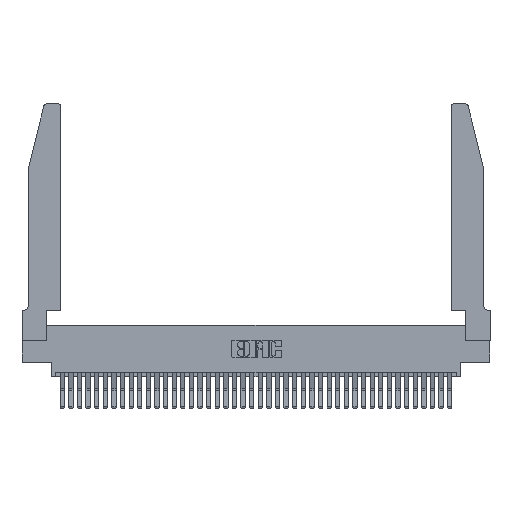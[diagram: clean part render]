
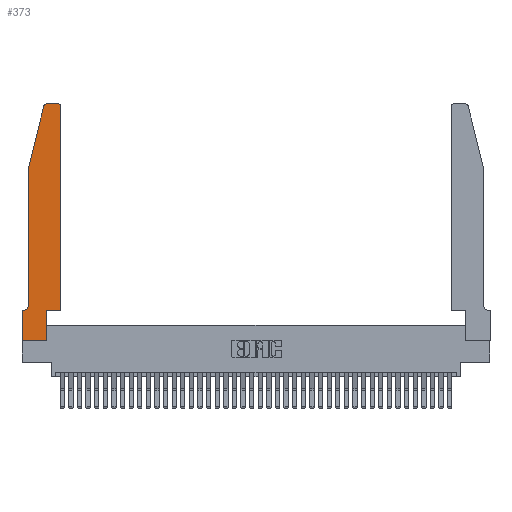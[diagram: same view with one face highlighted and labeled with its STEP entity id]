
A CAD part, top view. The second image highlights one B-rep face of the part: STEP entity #373.
In plain terms, the highlighted planar face has unit normal (0, 0, 1).
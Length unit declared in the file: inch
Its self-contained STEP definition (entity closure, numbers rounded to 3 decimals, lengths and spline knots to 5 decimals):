
#373 = ADVANCED_FACE ( 'NONE', ( #22306 ), #39974, .T. ) ;
#503 = DIRECTION ( 'NONE',  ( 0., 0., 1. ) ) ;
#1064 = ORIENTED_EDGE ( 'NONE', *, *, #20258, .T. ) ;
#1208 = AXIS2_PLACEMENT_3D ( 'NONE', #26135, #7357, #29238 ) ;
#1246 = EDGE_CURVE ( 'NONE', #1962, #23233, #16376, .T. ) ;
#1313 = CARTESIAN_POINT ( 'NONE',  ( 0.0755, 0.35, 0.37 ) ) ;
#1356 = EDGE_CURVE ( 'NONE', #24464, #34777, #13426, .T. ) ;
#1374 = DIRECTION ( 'NONE',  ( 0., 0., -1. ) ) ;
#1413 = EDGE_CURVE ( 'NONE', #3583, #27949, #17829, .T. ) ;
#1902 = VERTEX_POINT ( 'NONE', #19401 ) ;
#1962 = VERTEX_POINT ( 'NONE', #4251 ) ;
#2274 = LINE ( 'NONE', #35966, #11715 ) ;
#2526 = CARTESIAN_POINT ( 'NONE',  ( 0., 0.35, 0.37 ) ) ;
#3385 = CARTESIAN_POINT ( 'NONE',  ( 0.4205, 2.75, 0.37 ) ) ;
#3583 = VERTEX_POINT ( 'NONE', #28096 ) ;
#3814 = VERTEX_POINT ( 'NONE', #20504 ) ;
#4251 = CARTESIAN_POINT ( 'NONE',  ( 0.4505, 2.72, 0.37 ) ) ;
#4574 = EDGE_CURVE ( 'NONE', #27949, #27562, #8289, .T. ) ;
#4876 = VECTOR ( 'NONE', #6481, 39.37008 ) ;
#5573 = AXIS2_PLACEMENT_3D ( 'NONE', #20307, #1374, #23470 ) ;
#5749 = DIRECTION ( 'NONE',  ( 0., 0., 1. ) ) ;
#6366 = VECTOR ( 'NONE', #7573, 39.37008 ) ;
#6481 = DIRECTION ( 'NONE',  ( -0.239, -0.971, 0. ) ) ;
#6802 = VERTEX_POINT ( 'NONE', #23589 ) ;
#7245 = DIRECTION ( 'NONE',  ( 0., 1., 0. ) ) ;
#7311 = VECTOR ( 'NONE', #39691, 39.37008 ) ;
#7357 = DIRECTION ( 'NONE',  ( 0., 0., 1. ) ) ;
#7365 = LINE ( 'NONE', #20207, #6366 ) ;
#7573 = DIRECTION ( 'NONE',  ( -1., 0., 0. ) ) ;
#8111 = EDGE_CURVE ( 'NONE', #37173, #3814, #37953, .T. ) ;
#8289 = LINE ( 'NONE', #27271, #7311 ) ;
#9199 = CARTESIAN_POINT ( 'NONE',  ( 0.2865, 0.35, 0.37 ) ) ;
#9563 = ORIENTED_EDGE ( 'NONE', *, *, #8111, .T. ) ;
#9931 = CIRCLE ( 'NONE', #5573, 0.07 ) ;
#10021 = ORIENTED_EDGE ( 'NONE', *, *, #1356, .T. ) ;
#10969 = EDGE_CURVE ( 'NONE', #35680, #1962, #33832, .T. ) ;
#11715 = VECTOR ( 'NONE', #14183, 39.37008 ) ;
#12067 = EDGE_CURVE ( 'NONE', #34777, #1902, #19646, .T. ) ;
#12538 = CARTESIAN_POINT ( 'NONE',  ( 0.2865, 0., 0.37 ) ) ;
#12954 = VECTOR ( 'NONE', #15835, 39.37008 ) ;
#12986 = ORIENTED_EDGE ( 'NONE', *, *, #14734, .T. ) ;
#13120 = VECTOR ( 'NONE', #21284, 39.37008 ) ;
#13426 = CIRCLE ( 'NONE', #1208, 0.03 ) ;
#13847 = DIRECTION ( 'NONE',  ( 1., 0., 0. ) ) ;
#14183 = DIRECTION ( 'NONE',  ( 0., -1., 0. ) ) ;
#14216 = AXIS2_PLACEMENT_3D ( 'NONE', #2526, #5749, #27666 ) ;
#14734 = EDGE_CURVE ( 'NONE', #6802, #3583, #9931, .T. ) ;
#14781 = CARTESIAN_POINT ( 'NONE',  ( 0.284, 2.75, 0.37 ) ) ;
#15835 = DIRECTION ( 'NONE',  ( 1., 0., 0. ) ) ;
#15851 = CARTESIAN_POINT ( 'NONE',  ( 0.0755, 2., 0.37 ) ) ;
#16376 = CIRCLE ( 'NONE', #37693, 0.03 ) ;
#16624 = LINE ( 'NONE', #29404, #32203 ) ;
#16729 = CARTESIAN_POINT ( 'NONE',  ( 0.4505, 0.35, 0.37 ) ) ;
#17829 = LINE ( 'NONE', #1313, #26137 ) ;
#18476 = ORIENTED_EDGE ( 'NONE', *, *, #1246, .T. ) ;
#19401 = CARTESIAN_POINT ( 'NONE',  ( 0.0755, 2., 0.37 ) ) ;
#19414 = CARTESIAN_POINT ( 'NONE',  ( 0., 0., 0.37 ) ) ;
#19434 = CARTESIAN_POINT ( 'NONE',  ( 0.4205, 2.72, 0.37 ) ) ;
#19646 = LINE ( 'NONE', #15851, #4876 ) ;
#19858 = ORIENTED_EDGE ( 'NONE', *, *, #27042, .T. ) ;
#20207 = CARTESIAN_POINT ( 'NONE',  ( 0.2605, 2.75, 0.37 ) ) ;
#20258 = EDGE_CURVE ( 'NONE', #27562, #37173, #36812, .T. ) ;
#20307 = CARTESIAN_POINT ( 'NONE',  ( 0.0055, 0.42, 0.37 ) ) ;
#20334 = ORIENTED_EDGE ( 'NONE', *, *, #40394, .T. ) ;
#20504 = CARTESIAN_POINT ( 'NONE',  ( 0.2865, 0.35, 0.37 ) ) ;
#21284 = DIRECTION ( 'NONE',  ( 0., 1., 0. ) ) ;
#22306 = FACE_OUTER_BOUND ( 'NONE', #33698, .T. ) ;
#22613 = DIRECTION ( 'NONE',  ( 1., 0., 0. ) ) ;
#23233 = VERTEX_POINT ( 'NONE', #3385 ) ;
#23297 = ORIENTED_EDGE ( 'NONE', *, *, #1413, .T. ) ;
#23412 = DIRECTION ( 'NONE',  ( -1., 0., 0. ) ) ;
#23470 = DIRECTION ( 'NONE',  ( -1., 0., 0. ) ) ;
#23589 = CARTESIAN_POINT ( 'NONE',  ( 0.0755, 0.42, 0.37 ) ) ;
#23772 = ORIENTED_EDGE ( 'NONE', *, *, #32346, .T. ) ;
#24308 = CARTESIAN_POINT ( 'NONE',  ( 0.25487, 2.72718, 0.37 ) ) ;
#24464 = VERTEX_POINT ( 'NONE', #14781 ) ;
#26034 = CARTESIAN_POINT ( 'NONE',  ( 0.4505, 0.35, 0.37 ) ) ;
#26135 = CARTESIAN_POINT ( 'NONE',  ( 0.284, 2.72, 0.37 ) ) ;
#26137 = VECTOR ( 'NONE', #23412, 39.37008 ) ;
#26574 = VECTOR ( 'NONE', #7245, 39.37008 ) ;
#26670 = ORIENTED_EDGE ( 'NONE', *, *, #12067, .T. ) ;
#27042 = EDGE_CURVE ( 'NONE', #3814, #35680, #16624, .T. ) ;
#27271 = CARTESIAN_POINT ( 'NONE',  ( 0., 0., 0.37 ) ) ;
#27562 = VERTEX_POINT ( 'NONE', #19414 ) ;
#27666 = DIRECTION ( 'NONE',  ( 1., 0., 0. ) ) ;
#27949 = VERTEX_POINT ( 'NONE', #33385 ) ;
#28096 = CARTESIAN_POINT ( 'NONE',  ( 0.0055, 0.35, 0.37 ) ) ;
#28144 = ORIENTED_EDGE ( 'NONE', *, *, #10969, .T. ) ;
#29238 = DIRECTION ( 'NONE',  ( 1., 0., 0. ) ) ;
#29404 = CARTESIAN_POINT ( 'NONE',  ( 0.4505, 0.35, 0.37 ) ) ;
#32203 = VECTOR ( 'NONE', #13847, 39.37008 ) ;
#32346 = EDGE_CURVE ( 'NONE', #23233, #24464, #7365, .T. ) ;
#33385 = CARTESIAN_POINT ( 'NONE',  ( 0., 0.35, 0.37 ) ) ;
#33698 = EDGE_LOOP ( 'NONE', ( #23772, #10021, #26670, #20334, #12986, #23297, #39733, #1064, #9563, #19858, #28144, #18476 ) ) ;
#33832 = LINE ( 'NONE', #26034, #26574 ) ;
#34464 = CARTESIAN_POINT ( 'NONE',  ( 0., 0., 0.37 ) ) ;
#34777 = VERTEX_POINT ( 'NONE', #24308 ) ;
#35680 = VERTEX_POINT ( 'NONE', #16729 ) ;
#35966 = CARTESIAN_POINT ( 'NONE',  ( 0.0755, 2., 0.37 ) ) ;
#36812 = LINE ( 'NONE', #34464, #12954 ) ;
#37173 = VERTEX_POINT ( 'NONE', #12538 ) ;
#37693 = AXIS2_PLACEMENT_3D ( 'NONE', #19434, #503, #22613 ) ;
#37953 = LINE ( 'NONE', #9199, #13120 ) ;
#39691 = DIRECTION ( 'NONE',  ( 0., -1., 0. ) ) ;
#39733 = ORIENTED_EDGE ( 'NONE', *, *, #4574, .T. ) ;
#39974 = PLANE ( 'NONE',  #14216 ) ;
#40394 = EDGE_CURVE ( 'NONE', #1902, #6802, #2274, .T. ) ;
